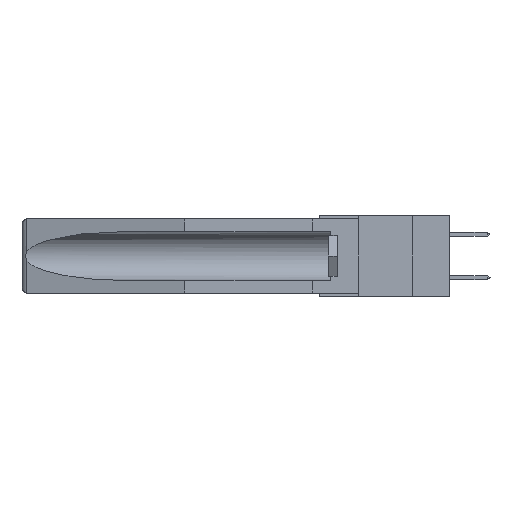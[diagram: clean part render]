
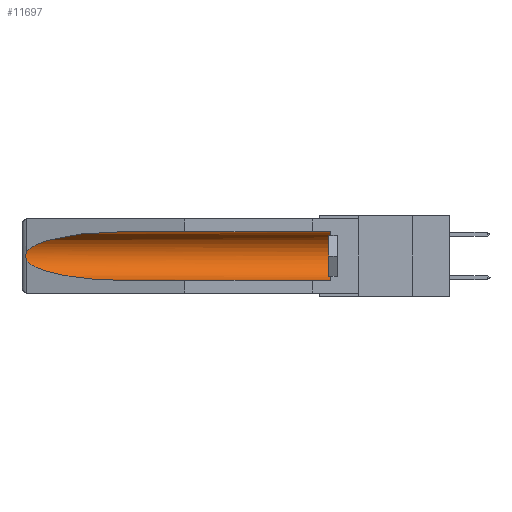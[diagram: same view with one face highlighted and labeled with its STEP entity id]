
A CAD part, left-side view. The second image highlights one B-rep face of the part: STEP entity #11697.
In plain terms, the highlighted cylindrical face has radius 2.857 mm (diameter 5.715 mm), a partial arc.
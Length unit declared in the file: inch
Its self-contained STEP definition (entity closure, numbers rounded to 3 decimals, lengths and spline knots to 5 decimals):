
#750 = CARTESIAN_POINT ( 'NONE',  ( 0.155, -0.30754, -0.284 ) ) ;
#1238 = VERTEX_POINT ( 'NONE', #4721 ) ;
#1264 = B_SPLINE_CURVE_WITH_KNOTS ( 'NONE', 3,
 ( #9792, #13772, #13663, #15010, #9938, #9846, #13559, #16339, #7313, #3441 ),
 .UNSPECIFIED., .F., .F.,
 ( 4, 2, 2, 2, 4 ),
 ( 0., 0.00029, 0.00058, 0.00087, 0.00117 ),
 .UNSPECIFIED. ) ;
#1431 = VERTEX_POINT ( 'NONE', #1478 ) ;
#1437 = EDGE_CURVE ( 'NONE', #1431, #3904, #3596, .T. ) ;
#1478 = CARTESIAN_POINT ( 'NONE',  ( 0.155, 0.126, -0.059 ) ) ;
#1667 = CARTESIAN_POINT ( 'NONE',  ( 0.155, 1.07973, -0.059 ) ) ;
#1668 = CARTESIAN_POINT ( 'NONE',  ( 0.26537, 1.52718, -0.14972 ) ) ;
#2023 = EDGE_CURVE ( 'NONE', #1238, #10916, #15760, .T. ) ;
#2388 = CARTESIAN_POINT ( 'NONE',  ( 0.26537, 1.52718, -0.19328 ) ) ;
#2552 = ORIENTED_EDGE ( 'NONE', *, *, #15479, .T. ) ;
#2901 = CARTESIAN_POINT ( 'NONE',  ( 0.155, 1.07973, -0.059 ) ) ;
#3441 = CARTESIAN_POINT ( 'NONE',  ( 0.26537, 1.52718, -0.19328 ) ) ;
#3596 = LINE ( 'NONE', #11824, #4814 ) ;
#3599 = VERTEX_POINT ( 'NONE', #10356 ) ;
#3904 = VERTEX_POINT ( 'NONE', #1667 ) ;
#3907 = VERTEX_POINT ( 'NONE', #15695 ) ;
#4039 = DIRECTION ( 'NONE',  ( 0., 1., 0. ) ) ;
#4288 = CARTESIAN_POINT ( 'NONE',  ( 0.21114, 1.30732, -0.059 ) ) ;
#4721 = CARTESIAN_POINT ( 'NONE',  ( 0.155, 0.126, -0.284 ) ) ;
#4744 = FACE_OUTER_BOUND ( 'NONE', #12822, .T. ) ;
#4814 = VECTOR ( 'NONE', #4039, 39.37008 ) ;
#5043 = EDGE_CURVE ( 'NONE', #3907, #3599, #1264, .T. ) ;
#5746 = DIRECTION ( 'NONE',  ( 0., 0., 1. ) ) ;
#5957 = DIRECTION ( 'NONE',  ( 0., 1., 0. ) ) ;
#6023 = AXIS2_PLACEMENT_3D ( 'NONE', #14527, #14591, #8251 ) ;
#6625 = AXIS2_PLACEMENT_3D ( 'NONE', #14717, #9548, #5746 ) ;
#7239 = ORIENTED_EDGE ( 'NONE', *, *, #12724, .T. ) ;
#7313 = CARTESIAN_POINT ( 'NONE',  ( 0.26597, 1.5296, -0.19026 ) ) ;
#7432 =( BOUNDED_CURVE ( )  B_SPLINE_CURVE ( 3, ( #2901, #4288, #8246, #1668 ),
 .UNSPECIFIED., .F., .F. ) 
 B_SPLINE_CURVE_WITH_KNOTS ( ( 4, 4 ),
 ( 4.71239, 6.08839 ),
 .UNSPECIFIED. ) 
 CURVE ( )  GEOMETRIC_REPRESENTATION_ITEM ( )  RATIONAL_B_SPLINE_CURVE ( ( 1., 0.848, 0.848, 1. ) ) 
 REPRESENTATION_ITEM ( '' )  );
#7529 = CIRCLE ( 'NONE', #6023, 0.1125 ) ;
#8114 = ORIENTED_EDGE ( 'NONE', *, *, #12254, .T. ) ;
#8146 = CARTESIAN_POINT ( 'NONE',  ( 0.155, 1.07973, -0.284 ) ) ;
#8246 = CARTESIAN_POINT ( 'NONE',  ( 0.25451, 1.48313, -0.09465 ) ) ;
#8251 = DIRECTION ( 'NONE',  ( 0., 0., 1. ) ) ;
#8677 =( BOUNDED_CURVE ( )  B_SPLINE_CURVE ( 3, ( #2388, #12475, #16409, #11323 ),
 .UNSPECIFIED., .F., .F. ) 
 B_SPLINE_CURVE_WITH_KNOTS ( ( 4, 4 ),
 ( 0.1948, 1.5708 ),
 .UNSPECIFIED. ) 
 CURVE ( )  GEOMETRIC_REPRESENTATION_ITEM ( )  RATIONAL_B_SPLINE_CURVE ( ( 1., 0.848, 0.848, 1. ) ) 
 REPRESENTATION_ITEM ( '' )  );
#8952 = CYLINDRICAL_SURFACE ( 'NONE', #6625, 0.1125 ) ;
#9548 = DIRECTION ( 'NONE',  ( 0., 1., 0. ) ) ;
#9792 = CARTESIAN_POINT ( 'NONE',  ( 0.26537, 1.52718, -0.14972 ) ) ;
#9846 = CARTESIAN_POINT ( 'NONE',  ( 0.2675, 1.53308, -0.17534 ) ) ;
#9938 = CARTESIAN_POINT ( 'NONE',  ( 0.2675, 1.53308, -0.16763 ) ) ;
#10356 = CARTESIAN_POINT ( 'NONE',  ( 0.26537, 1.52718, -0.19328 ) ) ;
#10916 = VERTEX_POINT ( 'NONE', #8146 ) ;
#11323 = CARTESIAN_POINT ( 'NONE',  ( 0.155, 1.07973, -0.284 ) ) ;
#11697 = ADVANCED_FACE ( 'NONE', ( #4744 ), #8952, .F. ) ;
#11824 = CARTESIAN_POINT ( 'NONE',  ( 0.155, -0.30754, -0.059 ) ) ;
#12254 = EDGE_CURVE ( 'NONE', #1238, #1431, #7529, .T. ) ;
#12309 = ORIENTED_EDGE ( 'NONE', *, *, #5043, .T. ) ;
#12404 = VECTOR ( 'NONE', #5957, 39.37008 ) ;
#12475 = CARTESIAN_POINT ( 'NONE',  ( 0.25451, 1.48313, -0.24835 ) ) ;
#12724 = EDGE_CURVE ( 'NONE', #3904, #3907, #7432, .T. ) ;
#12822 = EDGE_LOOP ( 'NONE', ( #7239, #12309, #2552, #15850, #8114, #13496 ) ) ;
#13496 = ORIENTED_EDGE ( 'NONE', *, *, #1437, .T. ) ;
#13559 = CARTESIAN_POINT ( 'NONE',  ( 0.2673, 1.53269, -0.17917 ) ) ;
#13663 = CARTESIAN_POINT ( 'NONE',  ( 0.26654, 1.53092, -0.15636 ) ) ;
#13772 = CARTESIAN_POINT ( 'NONE',  ( 0.26597, 1.52961, -0.15275 ) ) ;
#14527 = CARTESIAN_POINT ( 'NONE',  ( 0.155, 0.126, -0.1715 ) ) ;
#14591 = DIRECTION ( 'NONE',  ( 0., -1., 0. ) ) ;
#14717 = CARTESIAN_POINT ( 'NONE',  ( 0.155, -0.30754, -0.1715 ) ) ;
#15010 = CARTESIAN_POINT ( 'NONE',  ( 0.2673, 1.5327, -0.16383 ) ) ;
#15479 = EDGE_CURVE ( 'NONE', #3599, #10916, #8677, .T. ) ;
#15695 = CARTESIAN_POINT ( 'NONE',  ( 0.26537, 1.52718, -0.14972 ) ) ;
#15760 = LINE ( 'NONE', #750, #12404 ) ;
#15850 = ORIENTED_EDGE ( 'NONE', *, *, #2023, .F. ) ;
#16339 = CARTESIAN_POINT ( 'NONE',  ( 0.26655, 1.53094, -0.18657 ) ) ;
#16409 = CARTESIAN_POINT ( 'NONE',  ( 0.21114, 1.30732, -0.284 ) ) ;
